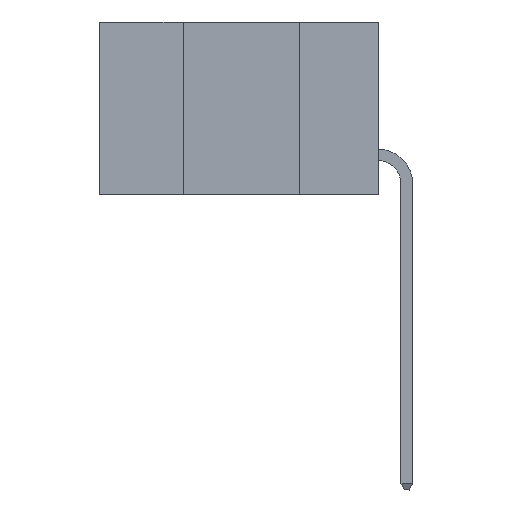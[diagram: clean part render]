
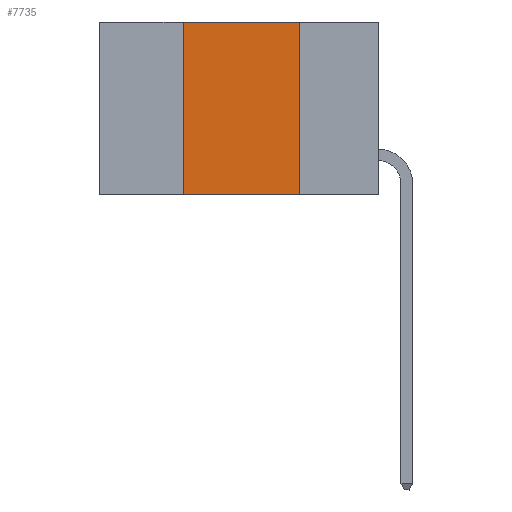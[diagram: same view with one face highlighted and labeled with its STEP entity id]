
A CAD part, left-side view. The second image highlights one B-rep face of the part: STEP entity #7735.
In plain terms, the highlighted planar face has unit normal (-1, 0, 0).
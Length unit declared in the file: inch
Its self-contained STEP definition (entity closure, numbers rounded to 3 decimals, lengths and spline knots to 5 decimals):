
#492 = VECTOR ( 'NONE', #2400, 39.37008 ) ;
#709 = EDGE_CURVE ( 'NONE', #1634, #6647, #1287, .T. ) ;
#884 = VERTEX_POINT ( 'NONE', #2416 ) ;
#1248 = DIRECTION ( 'NONE',  ( 0., -1., 0. ) ) ;
#1287 = LINE ( 'NONE', #5702, #1427 ) ;
#1427 = VECTOR ( 'NONE', #6596, 39.37008 ) ;
#1634 = VERTEX_POINT ( 'NONE', #6467 ) ;
#1923 = CARTESIAN_POINT ( 'NONE',  ( 0., 0.6, 0. ) ) ;
#2161 = VECTOR ( 'NONE', #2391, 39.37008 ) ;
#2180 = AXIS2_PLACEMENT_3D ( 'NONE', #5467, #2350, #2393 ) ;
#2350 = DIRECTION ( 'NONE',  ( 1., 0., 0. ) ) ;
#2391 = DIRECTION ( 'NONE',  ( 0., 0., 1. ) ) ;
#2393 = DIRECTION ( 'NONE',  ( 0., 0., -1. ) ) ;
#2400 = DIRECTION ( 'NONE',  ( 0., -1., 0. ) ) ;
#2416 = CARTESIAN_POINT ( 'NONE',  ( 0., 0.42, 0. ) ) ;
#2453 = ORIENTED_EDGE ( 'NONE', *, *, #8140, .F. ) ;
#2549 = PLANE ( 'NONE',  #2180 ) ;
#2647 = CARTESIAN_POINT ( 'NONE',  ( 0., 0.42, -0.37 ) ) ;
#3025 = ORIENTED_EDGE ( 'NONE', *, *, #709, .F. ) ;
#3091 = ORIENTED_EDGE ( 'NONE', *, *, #6390, .F. ) ;
#3197 = CARTESIAN_POINT ( 'NONE',  ( 0., 0.42, -0.37 ) ) ;
#3497 = LINE ( 'NONE', #1923, #3548 ) ;
#3542 = CARTESIAN_POINT ( 'NONE',  ( 0., 0.17, -0.37 ) ) ;
#3548 = VECTOR ( 'NONE', #1248, 39.37008 ) ;
#3690 = CARTESIAN_POINT ( 'NONE',  ( 0., 0.6, -0.37 ) ) ;
#4635 = VERTEX_POINT ( 'NONE', #2647 ) ;
#5467 = CARTESIAN_POINT ( 'NONE',  ( 0., 0.6, 0. ) ) ;
#5702 = CARTESIAN_POINT ( 'NONE',  ( 0., 0.17, -0.37 ) ) ;
#5713 = EDGE_CURVE ( 'NONE', #4635, #6647, #6630, .T. ) ;
#6237 = ORIENTED_EDGE ( 'NONE', *, *, #5713, .T. ) ;
#6390 = EDGE_CURVE ( 'NONE', #4635, #884, #8387, .T. ) ;
#6467 = CARTESIAN_POINT ( 'NONE',  ( 0., 0.17, 0. ) ) ;
#6596 = DIRECTION ( 'NONE',  ( 0., 0., -1. ) ) ;
#6630 = LINE ( 'NONE', #3690, #492 ) ;
#6647 = VERTEX_POINT ( 'NONE', #3542 ) ;
#6867 = FACE_OUTER_BOUND ( 'NONE', #9138, .T. ) ;
#7735 = ADVANCED_FACE ( 'NONE', ( #6867 ), #2549, .F. ) ;
#8140 = EDGE_CURVE ( 'NONE', #884, #1634, #3497, .T. ) ;
#8387 = LINE ( 'NONE', #3197, #2161 ) ;
#9138 = EDGE_LOOP ( 'NONE', ( #3025, #2453, #3091, #6237 ) ) ;
